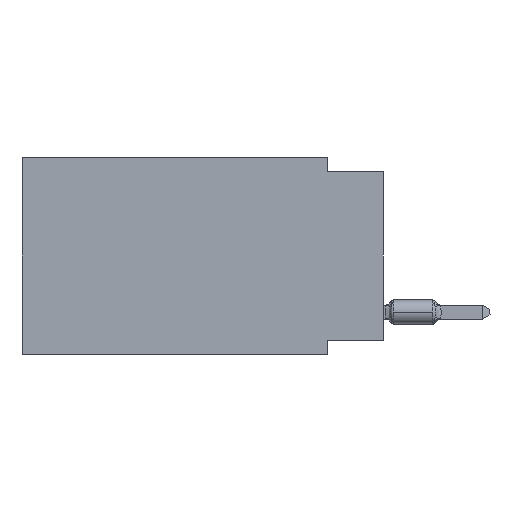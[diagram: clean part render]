
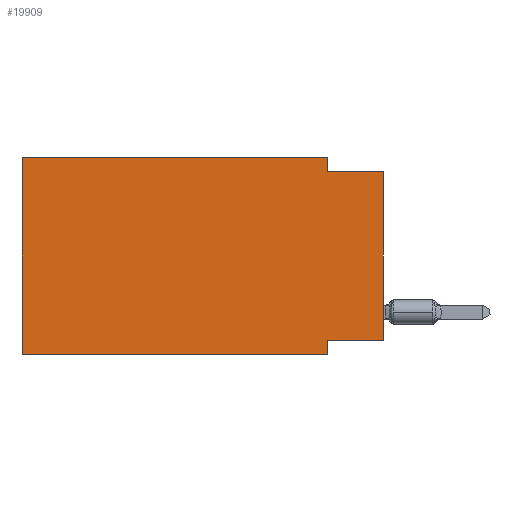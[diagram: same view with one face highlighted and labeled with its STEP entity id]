
A CAD part, left-side view. The second image highlights one B-rep face of the part: STEP entity #19909.
In plain terms, the highlighted planar face has unit normal (-1, 0, 0).
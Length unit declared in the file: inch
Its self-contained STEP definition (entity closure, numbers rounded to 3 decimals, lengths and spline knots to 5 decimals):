
#274 = CARTESIAN_POINT ( 'NONE',  ( 0., 0., -0.325 ) ) ;
#410 = CARTESIAN_POINT ( 'NONE',  ( 0., 0., -0.325 ) ) ;
#614 = CARTESIAN_POINT ( 'NONE',  ( 0., 0.645, -0.35 ) ) ;
#721 = CARTESIAN_POINT ( 'NONE',  ( 0., 0.1, -0.35 ) ) ;
#742 = ORIENTED_EDGE ( 'NONE', *, *, #5342, .T. ) ;
#1015 = DIRECTION ( 'NONE',  ( 0., -1., 0. ) ) ;
#1662 = CARTESIAN_POINT ( 'NONE',  ( 0., 0., -0.025 ) ) ;
#2030 = DIRECTION ( 'NONE',  ( 0., -1., 0. ) ) ;
#2108 = LINE ( 'NONE', #410, #5829 ) ;
#2165 = ORIENTED_EDGE ( 'NONE', *, *, #10735, .T. ) ;
#2661 = DIRECTION ( 'NONE',  ( 0., -1., 0. ) ) ;
#3332 = VECTOR ( 'NONE', #12711, 39.37008 ) ;
#3377 = EDGE_CURVE ( 'NONE', #23768, #7669, #14606, .T. ) ;
#3660 = AXIS2_PLACEMENT_3D ( 'NONE', #16013, #14431, #21816 ) ;
#4169 = VERTEX_POINT ( 'NONE', #12828 ) ;
#4196 = CARTESIAN_POINT ( 'NONE',  ( 0., 0.1, -0.025 ) ) ;
#4410 = EDGE_CURVE ( 'NONE', #10692, #18380, #10264, .T. ) ;
#4487 = ORIENTED_EDGE ( 'NONE', *, *, #14186, .F. ) ;
#5114 = VERTEX_POINT ( 'NONE', #274 ) ;
#5342 = EDGE_CURVE ( 'NONE', #5114, #17660, #20087, .T. ) ;
#5672 = ORIENTED_EDGE ( 'NONE', *, *, #16501, .F. ) ;
#5829 = VECTOR ( 'NONE', #15050, 39.37008 ) ;
#6146 = CARTESIAN_POINT ( 'NONE',  ( 0., 0.1, 0. ) ) ;
#7669 = VERTEX_POINT ( 'NONE', #20207 ) ;
#8077 = DIRECTION ( 'NONE',  ( 0., 0., -1. ) ) ;
#8679 = VECTOR ( 'NONE', #8789, 39.37008 ) ;
#8789 = DIRECTION ( 'NONE',  ( 0., 0., 1. ) ) ;
#8831 = CARTESIAN_POINT ( 'NONE',  ( 0., 0., 0. ) ) ;
#9057 = VECTOR ( 'NONE', #2661, 39.37008 ) ;
#9193 = ORIENTED_EDGE ( 'NONE', *, *, #3377, .F. ) ;
#9208 = CARTESIAN_POINT ( 'NONE',  ( 0., 0.1, -0.325 ) ) ;
#9652 = LINE ( 'NONE', #6146, #19803 ) ;
#10264 = LINE ( 'NONE', #721, #23409 ) ;
#10680 = PLANE ( 'NONE',  #3660 ) ;
#10692 = VERTEX_POINT ( 'NONE', #9208 ) ;
#10735 = EDGE_CURVE ( 'NONE', #23768, #18380, #13677, .T. ) ;
#11870 = ORIENTED_EDGE ( 'NONE', *, *, #14068, .F. ) ;
#12711 = DIRECTION ( 'NONE',  ( 0., 0., 1. ) ) ;
#12828 = CARTESIAN_POINT ( 'NONE',  ( 0., 0.1, 0. ) ) ;
#13677 = LINE ( 'NONE', #614, #9057 ) ;
#14068 = EDGE_CURVE ( 'NONE', #5114, #10692, #2108, .T. ) ;
#14186 = EDGE_CURVE ( 'NONE', #7669, #4169, #20383, .T. ) ;
#14431 = DIRECTION ( 'NONE',  ( 1., 0., 0. ) ) ;
#14606 = LINE ( 'NONE', #20046, #8679 ) ;
#15050 = DIRECTION ( 'NONE',  ( 0., 1., 0. ) ) ;
#15479 = DIRECTION ( 'NONE',  ( 0., 0., -1. ) ) ;
#16013 = CARTESIAN_POINT ( 'NONE',  ( 0., 0.645, 0. ) ) ;
#16425 = EDGE_CURVE ( 'NONE', #20553, #17660, #18493, .T. ) ;
#16501 = EDGE_CURVE ( 'NONE', #4169, #20553, #9652, .T. ) ;
#17595 = CARTESIAN_POINT ( 'NONE',  ( 0., 0.645, 0. ) ) ;
#17603 = ORIENTED_EDGE ( 'NONE', *, *, #16425, .F. ) ;
#17660 = VERTEX_POINT ( 'NONE', #20072 ) ;
#17711 = FACE_OUTER_BOUND ( 'NONE', #21564, .T. ) ;
#18380 = VERTEX_POINT ( 'NONE', #23890 ) ;
#18493 = LINE ( 'NONE', #1662, #22518 ) ;
#19803 = VECTOR ( 'NONE', #8077, 39.37008 ) ;
#19909 = ADVANCED_FACE ( 'NONE', ( #17711 ), #10680, .F. ) ;
#19912 = ORIENTED_EDGE ( 'NONE', *, *, #4410, .F. ) ;
#20046 = CARTESIAN_POINT ( 'NONE',  ( 0., 0.645, 0. ) ) ;
#20072 = CARTESIAN_POINT ( 'NONE',  ( 0., 0., -0.025 ) ) ;
#20087 = LINE ( 'NONE', #8831, #3332 ) ;
#20207 = CARTESIAN_POINT ( 'NONE',  ( 0., 0.645, 0. ) ) ;
#20383 = LINE ( 'NONE', #17595, #20900 ) ;
#20553 = VERTEX_POINT ( 'NONE', #4196 ) ;
#20900 = VECTOR ( 'NONE', #1015, 39.37008 ) ;
#21339 = CARTESIAN_POINT ( 'NONE',  ( 0., 0.645, -0.35 ) ) ;
#21564 = EDGE_LOOP ( 'NONE', ( #742, #17603, #5672, #4487, #9193, #2165, #19912, #11870 ) ) ;
#21816 = DIRECTION ( 'NONE',  ( 0., 0., -1. ) ) ;
#22518 = VECTOR ( 'NONE', #2030, 39.37008 ) ;
#23409 = VECTOR ( 'NONE', #15479, 39.37008 ) ;
#23768 = VERTEX_POINT ( 'NONE', #21339 ) ;
#23890 = CARTESIAN_POINT ( 'NONE',  ( 0., 0.1, -0.35 ) ) ;
